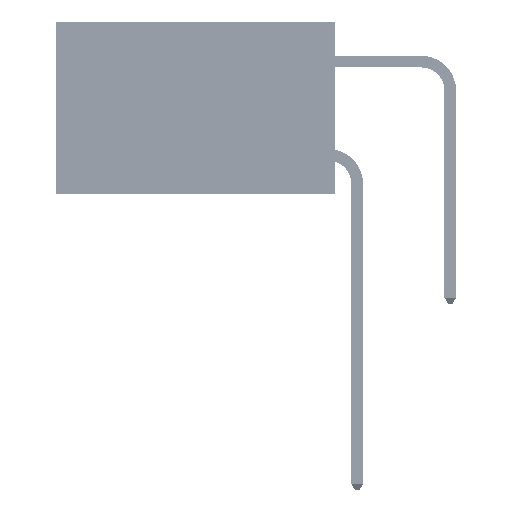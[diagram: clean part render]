
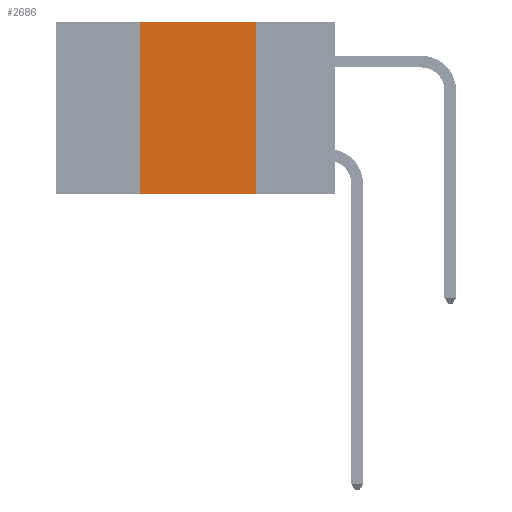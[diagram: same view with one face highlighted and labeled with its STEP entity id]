
A CAD part, left-side view. The second image highlights one B-rep face of the part: STEP entity #2686.
In plain terms, the highlighted planar face has unit normal (-1, 0, 0).
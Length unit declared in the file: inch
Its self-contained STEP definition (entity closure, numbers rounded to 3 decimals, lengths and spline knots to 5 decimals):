
#1319 = CARTESIAN_POINT ( 'NONE',  ( 0., 0.6, 0. ) ) ;
#1789 = VERTEX_POINT ( 'NONE', #48056 ) ;
#2319 = VERTEX_POINT ( 'NONE', #39611 ) ;
#2686 = ADVANCED_FACE ( 'NONE', ( #43916 ), #9223, .F. ) ;
#4008 = LINE ( 'NONE', #5033, #22543 ) ;
#5033 = CARTESIAN_POINT ( 'NONE',  ( 0., 0.42, 0. ) ) ;
#6469 = DIRECTION ( 'NONE',  ( 0., -1., 0. ) ) ;
#6528 = DIRECTION ( 'NONE',  ( 1., 0., 0. ) ) ;
#9223 = PLANE ( 'NONE',  #13701 ) ;
#12532 = VECTOR ( 'NONE', #6469, 39.37008 ) ;
#13358 = EDGE_CURVE ( 'NONE', #2319, #22929, #42283, .T. ) ;
#13536 = VECTOR ( 'NONE', #15510, 39.37008 ) ;
#13701 = AXIS2_PLACEMENT_3D ( 'NONE', #1319, #6528, #39147 ) ;
#14212 = LINE ( 'NONE', #29709, #26322 ) ;
#14987 = EDGE_CURVE ( 'NONE', #2319, #24794, #4008, .T. ) ;
#15510 = DIRECTION ( 'NONE',  ( 0., -1., 0. ) ) ;
#16229 = ORIENTED_EDGE ( 'NONE', *, *, #20453, .F. ) ;
#20178 = LINE ( 'NONE', #31061, #12532 ) ;
#20453 = EDGE_CURVE ( 'NONE', #24794, #1789, #20178, .T. ) ;
#22493 = EDGE_CURVE ( 'NONE', #1789, #22929, #14212, .T. ) ;
#22543 = VECTOR ( 'NONE', #46205, 39.37008 ) ;
#22929 = VERTEX_POINT ( 'NONE', #24667 ) ;
#23189 = CARTESIAN_POINT ( 'NONE',  ( 0., 0.6, -0.37 ) ) ;
#23438 = ORIENTED_EDGE ( 'NONE', *, *, #13358, .T. ) ;
#24667 = CARTESIAN_POINT ( 'NONE',  ( 0., 0.17, -0.37 ) ) ;
#24794 = VERTEX_POINT ( 'NONE', #43991 ) ;
#26322 = VECTOR ( 'NONE', #50401, 39.37008 ) ;
#29709 = CARTESIAN_POINT ( 'NONE',  ( 0., 0.17, 0. ) ) ;
#31061 = CARTESIAN_POINT ( 'NONE',  ( 0., 0.6, 0. ) ) ;
#35731 = EDGE_LOOP ( 'NONE', ( #48616, #16229, #48129, #23438 ) ) ;
#39147 = DIRECTION ( 'NONE',  ( 0., 0., -1. ) ) ;
#39611 = CARTESIAN_POINT ( 'NONE',  ( 0., 0.42, -0.37 ) ) ;
#42283 = LINE ( 'NONE', #23189, #13536 ) ;
#43916 = FACE_OUTER_BOUND ( 'NONE', #35731, .T. ) ;
#43991 = CARTESIAN_POINT ( 'NONE',  ( 0., 0.42, 0. ) ) ;
#46205 = DIRECTION ( 'NONE',  ( 0., 0., 1. ) ) ;
#48056 = CARTESIAN_POINT ( 'NONE',  ( 0., 0.17, 0. ) ) ;
#48129 = ORIENTED_EDGE ( 'NONE', *, *, #14987, .F. ) ;
#48616 = ORIENTED_EDGE ( 'NONE', *, *, #22493, .F. ) ;
#50401 = DIRECTION ( 'NONE',  ( 0., 0., -1. ) ) ;
